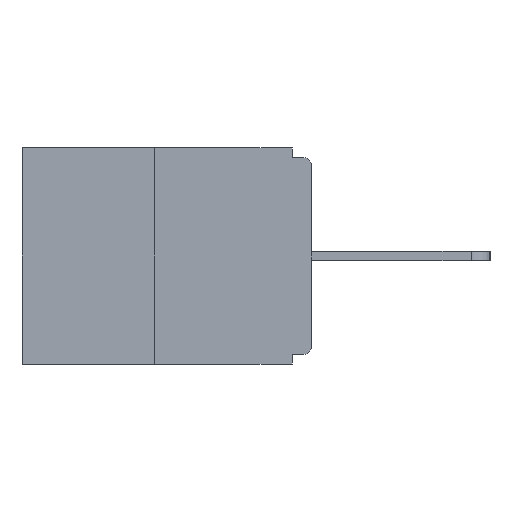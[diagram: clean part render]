
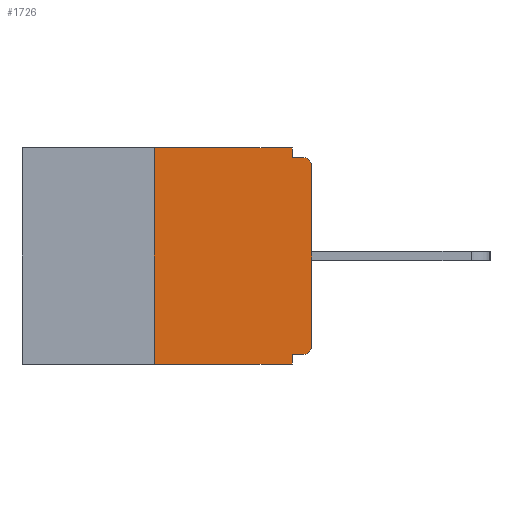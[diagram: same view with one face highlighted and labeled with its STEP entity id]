
A CAD part, left-side view. The second image highlights one B-rep face of the part: STEP entity #1726.
In plain terms, the highlighted planar face has unit normal (-1, 0, 0).
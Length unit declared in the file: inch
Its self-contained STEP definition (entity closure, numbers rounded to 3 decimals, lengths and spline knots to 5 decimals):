
#17 = DIRECTION ( 'NONE',  ( 0., -1., 0. ) ) ;
#1096 = ORIENTED_EDGE ( 'NONE', *, *, #15627, .F. ) ;
#1322 = ORIENTED_EDGE ( 'NONE', *, *, #9179, .T. ) ;
#1406 = EDGE_CURVE ( 'NONE', #11694, #19632, #12611, .T. ) ;
#1463 = ORIENTED_EDGE ( 'NONE', *, *, #12427, .F. ) ;
#1726 = ADVANCED_FACE ( 'NONE', ( #1923 ), #11490, .F. ) ;
#1923 = FACE_OUTER_BOUND ( 'NONE', #2514, .T. ) ;
#2017 = CARTESIAN_POINT ( 'NONE',  ( 0., 0.031, -0.328 ) ) ;
#2479 = LINE ( 'NONE', #17660, #13963 ) ;
#2514 = EDGE_LOOP ( 'NONE', ( #16164, #6386, #7879, #1463, #9890, #14868, #16752, #1322, #3927, #1096 ) ) ;
#3083 = CARTESIAN_POINT ( 'NONE',  ( 0., 0.031, 0. ) ) ;
#3350 = VERTEX_POINT ( 'NONE', #18795 ) ;
#3517 = VECTOR ( 'NONE', #9437, 39.37008 ) ;
#3665 = EDGE_CURVE ( 'NONE', #6012, #11965, #8856, .T. ) ;
#3927 = ORIENTED_EDGE ( 'NONE', *, *, #17593, .F. ) ;
#4033 = DIRECTION ( 'NONE',  ( 0., 0., -1. ) ) ;
#4436 = CARTESIAN_POINT ( 'NONE',  ( 0., 0.46, -0.343 ) ) ;
#5241 = LINE ( 'NONE', #7684, #9114 ) ;
#5585 = CARTESIAN_POINT ( 'NONE',  ( 0., 0.031, 0. ) ) ;
#5650 = LINE ( 'NONE', #20649, #9284 ) ;
#6012 = VERTEX_POINT ( 'NONE', #6940 ) ;
#6016 = LINE ( 'NONE', #5585, #9923 ) ;
#6386 = ORIENTED_EDGE ( 'NONE', *, *, #20813, .F. ) ;
#6940 = CARTESIAN_POINT ( 'NONE',  ( 0., 0., -0.313 ) ) ;
#7124 = VECTOR ( 'NONE', #8012, 39.37008 ) ;
#7547 = AXIS2_PLACEMENT_3D ( 'NONE', #20376, #10455, #17054 ) ;
#7684 = CARTESIAN_POINT ( 'NONE',  ( 0., 0., -0.328 ) ) ;
#7879 = ORIENTED_EDGE ( 'NONE', *, *, #14505, .T. ) ;
#8012 = DIRECTION ( 'NONE',  ( 0., -1., 0. ) ) ;
#8364 = DIRECTION ( 'NONE',  ( 0., 0., 1. ) ) ;
#8522 = CARTESIAN_POINT ( 'NONE',  ( 0., 0.015, -0.328 ) ) ;
#8572 = CARTESIAN_POINT ( 'NONE',  ( 0., 0., -0.03 ) ) ;
#8856 = LINE ( 'NONE', #21607, #21191 ) ;
#8959 = LINE ( 'NONE', #14404, #3517 ) ;
#9114 = VECTOR ( 'NONE', #19303, 39.37008 ) ;
#9179 = EDGE_CURVE ( 'NONE', #11965, #21421, #13361, .T. ) ;
#9209 = VERTEX_POINT ( 'NONE', #2017 ) ;
#9284 = VECTOR ( 'NONE', #13950, 39.37008 ) ;
#9308 = DIRECTION ( 'NONE',  ( 0., 0., -1. ) ) ;
#9437 = DIRECTION ( 'NONE',  ( 0., 0., 1. ) ) ;
#9619 = EDGE_CURVE ( 'NONE', #20459, #9209, #5241, .T. ) ;
#9890 = ORIENTED_EDGE ( 'NONE', *, *, #9619, .F. ) ;
#9923 = VECTOR ( 'NONE', #4033, 39.37008 ) ;
#10333 = CIRCLE ( 'NONE', #21183, 0.015 ) ;
#10455 = DIRECTION ( 'NONE',  ( -1., 0., 0. ) ) ;
#11221 = VERTEX_POINT ( 'NONE', #19955 ) ;
#11272 = CARTESIAN_POINT ( 'NONE',  ( 0., 0.46, 0. ) ) ;
#11490 = PLANE ( 'NONE',  #18516 ) ;
#11525 = CARTESIAN_POINT ( 'NONE',  ( 0., 0.031, -0.015 ) ) ;
#11694 = VERTEX_POINT ( 'NONE', #20908 ) ;
#11895 = CARTESIAN_POINT ( 'NONE',  ( 0., 0.015, -0.313 ) ) ;
#11965 = VERTEX_POINT ( 'NONE', #8572 ) ;
#12427 = EDGE_CURVE ( 'NONE', #9209, #3350, #2479, .T. ) ;
#12611 = LINE ( 'NONE', #20027, #19450 ) ;
#12855 = LINE ( 'NONE', #4436, #7124 ) ;
#13211 = CARTESIAN_POINT ( 'NONE',  ( 0., 0.015, -0.015 ) ) ;
#13361 = CIRCLE ( 'NONE', #7547, 0.015 ) ;
#13931 = VERTEX_POINT ( 'NONE', #11525 ) ;
#13950 = DIRECTION ( 'NONE',  ( 0., -1., 0. ) ) ;
#13963 = VECTOR ( 'NONE', #9308, 39.37008 ) ;
#14404 = CARTESIAN_POINT ( 'NONE',  ( 0., 0.25, 0. ) ) ;
#14505 = EDGE_CURVE ( 'NONE', #11221, #3350, #12855, .T. ) ;
#14634 = DIRECTION ( 'NONE',  ( 0., 0., -1. ) ) ;
#14868 = ORIENTED_EDGE ( 'NONE', *, *, #18018, .T. ) ;
#15627 = EDGE_CURVE ( 'NONE', #19632, #13931, #6016, .T. ) ;
#16164 = ORIENTED_EDGE ( 'NONE', *, *, #1406, .F. ) ;
#16752 = ORIENTED_EDGE ( 'NONE', *, *, #3665, .T. ) ;
#16965 = DIRECTION ( 'NONE',  ( 0., 0., -1. ) ) ;
#17054 = DIRECTION ( 'NONE',  ( 0., 0., -1. ) ) ;
#17593 = EDGE_CURVE ( 'NONE', #13931, #21421, #5650, .T. ) ;
#17660 = CARTESIAN_POINT ( 'NONE',  ( 0., 0.031, -0.343 ) ) ;
#18018 = EDGE_CURVE ( 'NONE', #20459, #6012, #10333, .T. ) ;
#18516 = AXIS2_PLACEMENT_3D ( 'NONE', #11272, #21406, #14634 ) ;
#18795 = CARTESIAN_POINT ( 'NONE',  ( 0., 0.031, -0.343 ) ) ;
#18808 = DIRECTION ( 'NONE',  ( -1., 0., 0. ) ) ;
#19303 = DIRECTION ( 'NONE',  ( 0., 1., 0. ) ) ;
#19450 = VECTOR ( 'NONE', #17, 39.37008 ) ;
#19632 = VERTEX_POINT ( 'NONE', #3083 ) ;
#19955 = CARTESIAN_POINT ( 'NONE',  ( 0., 0.25, -0.343 ) ) ;
#20027 = CARTESIAN_POINT ( 'NONE',  ( 0., 0.46, 0. ) ) ;
#20376 = CARTESIAN_POINT ( 'NONE',  ( 0., 0.015, -0.03 ) ) ;
#20459 = VERTEX_POINT ( 'NONE', #8522 ) ;
#20649 = CARTESIAN_POINT ( 'NONE',  ( 0., 0., -0.015 ) ) ;
#20813 = EDGE_CURVE ( 'NONE', #11221, #11694, #8959, .T. ) ;
#20908 = CARTESIAN_POINT ( 'NONE',  ( 0., 0.25, 0. ) ) ;
#21183 = AXIS2_PLACEMENT_3D ( 'NONE', #11895, #18808, #16965 ) ;
#21191 = VECTOR ( 'NONE', #8364, 39.37008 ) ;
#21406 = DIRECTION ( 'NONE',  ( 1., 0., 0. ) ) ;
#21421 = VERTEX_POINT ( 'NONE', #13211 ) ;
#21607 = CARTESIAN_POINT ( 'NONE',  ( 0., 0., 0. ) ) ;
